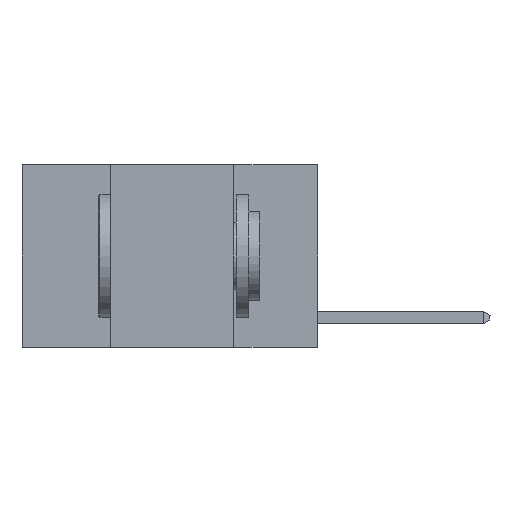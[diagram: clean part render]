
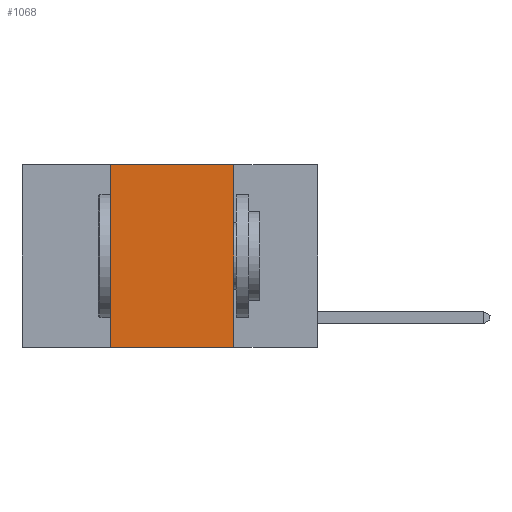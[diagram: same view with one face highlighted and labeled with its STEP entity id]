
A CAD part, left-side view. The second image highlights one B-rep face of the part: STEP entity #1068.
In plain terms, the highlighted planar face has unit normal (-1, 0, 0).
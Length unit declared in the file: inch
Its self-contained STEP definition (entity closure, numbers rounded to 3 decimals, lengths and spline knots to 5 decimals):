
#24 = DIRECTION ( 'NONE',  ( 0., 0., 1. ) ) ;
#480 = VERTEX_POINT ( 'NONE', #1156 ) ;
#1068 = ADVANCED_FACE ( 'NONE', ( #16304 ), #13273, .F. ) ;
#1156 = CARTESIAN_POINT ( 'NONE',  ( 0., 0.42, -0.37 ) ) ;
#2185 = CARTESIAN_POINT ( 'NONE',  ( 0., 0.17, 0. ) ) ;
#2697 = CARTESIAN_POINT ( 'NONE',  ( 0., 0.42, 0. ) ) ;
#3201 = VECTOR ( 'NONE', #24, 39.37008 ) ;
#3442 = DIRECTION ( 'NONE',  ( 0., -1., 0. ) ) ;
#3653 = LINE ( 'NONE', #16795, #3201 ) ;
#4000 = VECTOR ( 'NONE', #3442, 39.37008 ) ;
#4180 = CARTESIAN_POINT ( 'NONE',  ( 0., 0.17, -0.37 ) ) ;
#4702 = EDGE_CURVE ( 'NONE', #480, #15299, #3653, .T. ) ;
#5087 = VERTEX_POINT ( 'NONE', #2185 ) ;
#5610 = DIRECTION ( 'NONE',  ( 0., -1., 0. ) ) ;
#6696 = EDGE_CURVE ( 'NONE', #15299, #5087, #13324, .T. ) ;
#8177 = EDGE_CURVE ( 'NONE', #480, #8551, #11113, .T. ) ;
#8551 = VERTEX_POINT ( 'NONE', #4180 ) ;
#8573 = DIRECTION ( 'NONE',  ( 1., 0., 0. ) ) ;
#8916 = EDGE_CURVE ( 'NONE', #5087, #8551, #14120, .T. ) ;
#9053 = DIRECTION ( 'NONE',  ( 0., 0., -1. ) ) ;
#9241 = CARTESIAN_POINT ( 'NONE',  ( 0., 0.6, 0. ) ) ;
#9294 = EDGE_LOOP ( 'NONE', ( #13001, #13283, #13737, #14429 ) ) ;
#10833 = DIRECTION ( 'NONE',  ( 0., 0., -1. ) ) ;
#11113 = LINE ( 'NONE', #11926, #4000 ) ;
#11926 = CARTESIAN_POINT ( 'NONE',  ( 0., 0.6, -0.37 ) ) ;
#12656 = CARTESIAN_POINT ( 'NONE',  ( 0., 0.6, 0. ) ) ;
#12708 = AXIS2_PLACEMENT_3D ( 'NONE', #9241, #8573, #9053 ) ;
#13001 = ORIENTED_EDGE ( 'NONE', *, *, #8916, .F. ) ;
#13273 = PLANE ( 'NONE',  #12708 ) ;
#13283 = ORIENTED_EDGE ( 'NONE', *, *, #6696, .F. ) ;
#13324 = LINE ( 'NONE', #12656, #16980 ) ;
#13685 = VECTOR ( 'NONE', #10833, 39.37008 ) ;
#13737 = ORIENTED_EDGE ( 'NONE', *, *, #4702, .F. ) ;
#14120 = LINE ( 'NONE', #17695, #13685 ) ;
#14429 = ORIENTED_EDGE ( 'NONE', *, *, #8177, .T. ) ;
#15299 = VERTEX_POINT ( 'NONE', #2697 ) ;
#16304 = FACE_OUTER_BOUND ( 'NONE', #9294, .T. ) ;
#16795 = CARTESIAN_POINT ( 'NONE',  ( 0., 0.42, 0. ) ) ;
#16980 = VECTOR ( 'NONE', #5610, 39.37008 ) ;
#17695 = CARTESIAN_POINT ( 'NONE',  ( 0., 0.17, 0. ) ) ;
